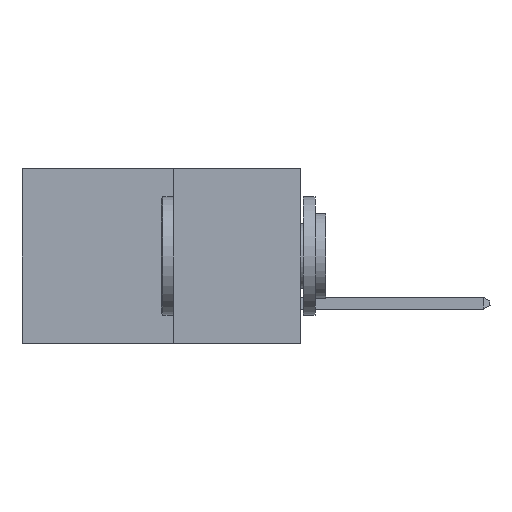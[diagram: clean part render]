
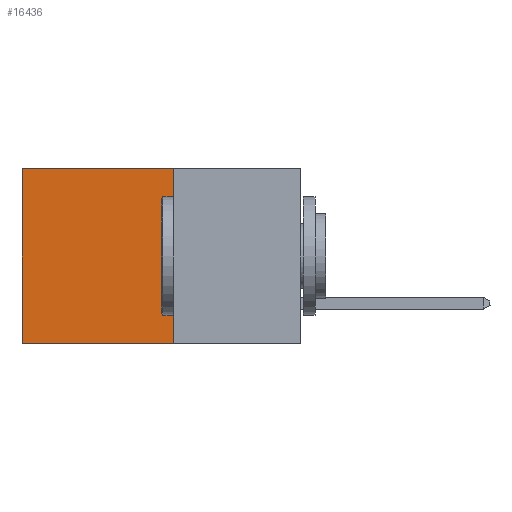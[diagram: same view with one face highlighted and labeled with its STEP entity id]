
A CAD part, left-side view. The second image highlights one B-rep face of the part: STEP entity #16436.
In plain terms, the highlighted planar face has unit normal (-1, 0, 0).
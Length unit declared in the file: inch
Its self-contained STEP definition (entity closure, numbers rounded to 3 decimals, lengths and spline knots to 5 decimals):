
#305 = CARTESIAN_POINT ( 'NONE',  ( 0.277, 0.27, -0.37 ) ) ;
#2054 = CARTESIAN_POINT ( 'NONE',  ( 0.277, 0.27, 0. ) ) ;
#2174 = DIRECTION ( 'NONE',  ( 1., 0., 0. ) ) ;
#2869 = VECTOR ( 'NONE', #14472, 39.37008 ) ;
#3447 = FACE_OUTER_BOUND ( 'NONE', #6340, .T. ) ;
#4034 = DIRECTION ( 'NONE',  ( 0., 0., -1. ) ) ;
#5698 = VERTEX_POINT ( 'NONE', #2054 ) ;
#5839 = PLANE ( 'NONE',  #10098 ) ;
#6073 = VERTEX_POINT ( 'NONE', #16227 ) ;
#6093 = VECTOR ( 'NONE', #4034, 39.37008 ) ;
#6340 = EDGE_LOOP ( 'NONE', ( #11217, #13022, #13829, #7230 ) ) ;
#7230 = ORIENTED_EDGE ( 'NONE', *, *, #12759, .T. ) ;
#7610 = CARTESIAN_POINT ( 'NONE',  ( 0.277, 0.59, 0. ) ) ;
#8192 = DIRECTION ( 'NONE',  ( 0., 1., 0. ) ) ;
#8531 = LINE ( 'NONE', #18999, #17968 ) ;
#10098 = AXIS2_PLACEMENT_3D ( 'NONE', #13406, #2174, #15302 ) ;
#10155 = CARTESIAN_POINT ( 'NONE',  ( 0.277, 0.59, -0.37 ) ) ;
#10389 = VERTEX_POINT ( 'NONE', #10155 ) ;
#10499 = LINE ( 'NONE', #305, #6093 ) ;
#11217 = ORIENTED_EDGE ( 'NONE', *, *, #15456, .T. ) ;
#12759 = EDGE_CURVE ( 'NONE', #5698, #22833, #8531, .T. ) ;
#13022 = ORIENTED_EDGE ( 'NONE', *, *, #21431, .F. ) ;
#13406 = CARTESIAN_POINT ( 'NONE',  ( 0.277, 0.27, -0.37 ) ) ;
#13829 = ORIENTED_EDGE ( 'NONE', *, *, #15119, .F. ) ;
#14472 = DIRECTION ( 'NONE',  ( 0., 0., -1. ) ) ;
#15119 = EDGE_CURVE ( 'NONE', #5698, #6073, #10499, .T. ) ;
#15302 = DIRECTION ( 'NONE',  ( 0., 0., -1. ) ) ;
#15456 = EDGE_CURVE ( 'NONE', #22833, #10389, #17849, .T. ) ;
#16227 = CARTESIAN_POINT ( 'NONE',  ( 0.277, 0.27, -0.37 ) ) ;
#16436 = ADVANCED_FACE ( 'NONE', ( #3447 ), #5839, .F. ) ;
#17849 = LINE ( 'NONE', #20143, #2869 ) ;
#17968 = VECTOR ( 'NONE', #20873, 39.37008 ) ;
#18999 = CARTESIAN_POINT ( 'NONE',  ( 0.277, 0.27, 0. ) ) ;
#20143 = CARTESIAN_POINT ( 'NONE',  ( 0.277, 0.59, -0.37 ) ) ;
#20621 = VECTOR ( 'NONE', #8192, 39.37008 ) ;
#20873 = DIRECTION ( 'NONE',  ( 0., 1., 0. ) ) ;
#21431 = EDGE_CURVE ( 'NONE', #6073, #10389, #21817, .T. ) ;
#21817 = LINE ( 'NONE', #23232, #20621 ) ;
#22833 = VERTEX_POINT ( 'NONE', #7610 ) ;
#23232 = CARTESIAN_POINT ( 'NONE',  ( 0.277, 0.27, -0.37 ) ) ;
